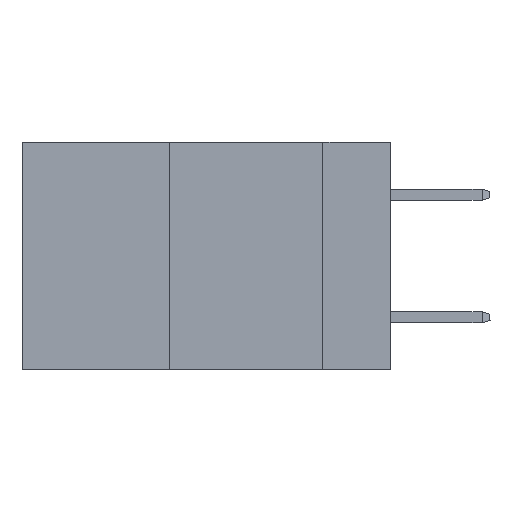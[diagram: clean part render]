
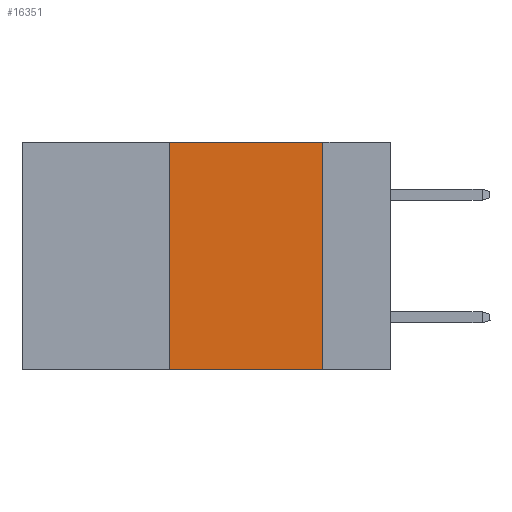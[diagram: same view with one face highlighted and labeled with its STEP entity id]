
A CAD part, left-side view. The second image highlights one B-rep face of the part: STEP entity #16351.
In plain terms, the highlighted planar face has unit normal (-1, 0, 0).
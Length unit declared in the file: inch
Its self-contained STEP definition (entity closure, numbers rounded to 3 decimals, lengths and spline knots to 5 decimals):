
#108 = VERTEX_POINT ( 'NONE', #15964 ) ;
#1846 = CARTESIAN_POINT ( 'NONE',  ( 0., 0.6, 0. ) ) ;
#2009 = LINE ( 'NONE', #11815, #2045 ) ;
#2045 = VECTOR ( 'NONE', #23800, 39.37008 ) ;
#2287 = DIRECTION ( 'NONE',  ( 0., 0., -1. ) ) ;
#4513 = ORIENTED_EDGE ( 'NONE', *, *, #23815, .F. ) ;
#4727 = LINE ( 'NONE', #1846, #7339 ) ;
#7144 = DIRECTION ( 'NONE',  ( 0., -1., 0. ) ) ;
#7339 = VECTOR ( 'NONE', #7144, 39.37008 ) ;
#7703 = EDGE_CURVE ( 'NONE', #23143, #20045, #19278, .T. ) ;
#9604 = VECTOR ( 'NONE', #2287, 39.37008 ) ;
#11701 = ORIENTED_EDGE ( 'NONE', *, *, #7703, .F. ) ;
#11815 = CARTESIAN_POINT ( 'NONE',  ( 0., 0.36, 0. ) ) ;
#12346 = EDGE_CURVE ( 'NONE', #28637, #20045, #22002, .T. ) ;
#14797 = CARTESIAN_POINT ( 'NONE',  ( 0., 0.6, -0.37 ) ) ;
#15332 = PLANE ( 'NONE',  #17144 ) ;
#15964 = CARTESIAN_POINT ( 'NONE',  ( 0., 0.36, 0. ) ) ;
#16351 = ADVANCED_FACE ( 'NONE', ( #27356 ), #15332, .F. ) ;
#17132 = ORIENTED_EDGE ( 'NONE', *, *, #29460, .F. ) ;
#17144 = AXIS2_PLACEMENT_3D ( 'NONE', #29751, #17411, #26896 ) ;
#17411 = DIRECTION ( 'NONE',  ( 1., 0., 0. ) ) ;
#18225 = CARTESIAN_POINT ( 'NONE',  ( 0., 0.11, 0. ) ) ;
#19278 = LINE ( 'NONE', #24249, #9604 ) ;
#19986 = EDGE_LOOP ( 'NONE', ( #11701, #17132, #4513, #28675 ) ) ;
#20045 = VERTEX_POINT ( 'NONE', #21178 ) ;
#21178 = CARTESIAN_POINT ( 'NONE',  ( 0., 0.11, -0.37 ) ) ;
#21672 = DIRECTION ( 'NONE',  ( 0., -1., 0. ) ) ;
#22002 = LINE ( 'NONE', #14797, #29326 ) ;
#23143 = VERTEX_POINT ( 'NONE', #18225 ) ;
#23800 = DIRECTION ( 'NONE',  ( 0., 0., 1. ) ) ;
#23815 = EDGE_CURVE ( 'NONE', #28637, #108, #2009, .T. ) ;
#24249 = CARTESIAN_POINT ( 'NONE',  ( 0., 0.11, 0. ) ) ;
#26896 = DIRECTION ( 'NONE',  ( 0., 0., -1. ) ) ;
#27356 = FACE_OUTER_BOUND ( 'NONE', #19986, .T. ) ;
#28565 = CARTESIAN_POINT ( 'NONE',  ( 0., 0.36, -0.37 ) ) ;
#28637 = VERTEX_POINT ( 'NONE', #28565 ) ;
#28675 = ORIENTED_EDGE ( 'NONE', *, *, #12346, .T. ) ;
#29326 = VECTOR ( 'NONE', #21672, 39.37008 ) ;
#29460 = EDGE_CURVE ( 'NONE', #108, #23143, #4727, .T. ) ;
#29751 = CARTESIAN_POINT ( 'NONE',  ( 0., 0.6, 0. ) ) ;
